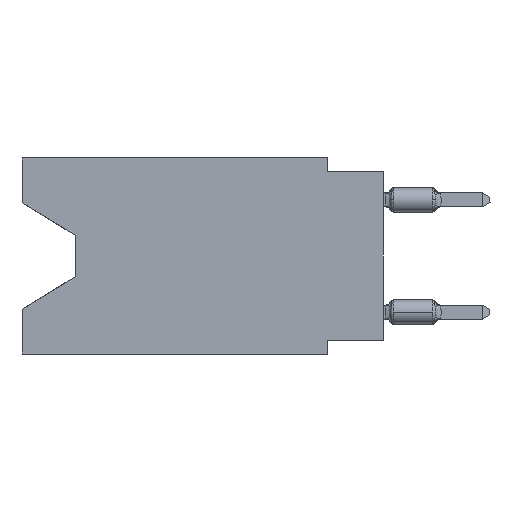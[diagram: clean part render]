
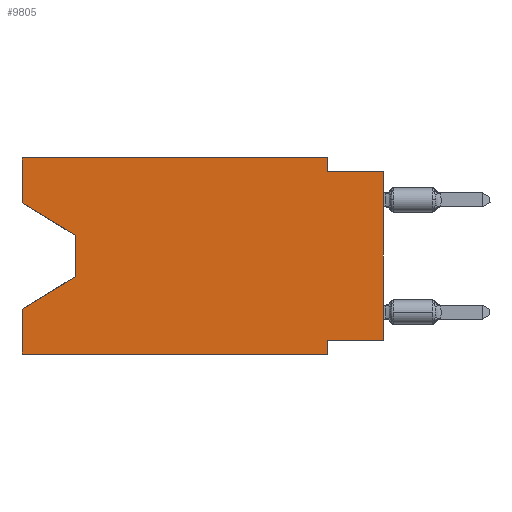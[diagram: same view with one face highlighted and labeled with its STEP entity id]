
A CAD part, left-side view. The second image highlights one B-rep face of the part: STEP entity #9805.
In plain terms, the highlighted planar face has unit normal (-1, 0, 0).
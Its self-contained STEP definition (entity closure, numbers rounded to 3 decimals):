
#19 = DIRECTION ( 'NONE',  ( 0., 0., 1. ) ) ;
#426 = EDGE_CURVE ( 'NONE', #23437, #9817, #18865, .T. ) ;
#440 = VECTOR ( 'NONE', #19, 1000. ) ;
#772 = EDGE_CURVE ( 'NONE', #21049, #9817, #8715, .T. ) ;
#2293 = ORIENTED_EDGE ( 'NONE', *, *, #16511, .F. ) ;
#2346 = ORIENTED_EDGE ( 'NONE', *, *, #4316, .F. ) ;
#2746 = DIRECTION ( 'NONE',  ( 0., 0., 1. ) ) ;
#3566 = ORIENTED_EDGE ( 'NONE', *, *, #21215, .T. ) ;
#3911 = PLANE ( 'NONE',  #6293 ) ;
#4005 = VERTEX_POINT ( 'NONE', #13388 ) ;
#4132 = CARTESIAN_POINT ( 'NONE',  ( 0., 16.383, -8.89 ) ) ;
#4316 = EDGE_CURVE ( 'NONE', #16762, #10100, #15087, .T. ) ;
#4825 = LINE ( 'NONE', #24658, #16931 ) ;
#5065 = CARTESIAN_POINT ( 'NONE',  ( 0., 2.54, -8.89 ) ) ;
#5200 = CARTESIAN_POINT ( 'NONE',  ( 0., 16.383, -8.89 ) ) ;
#5883 = CARTESIAN_POINT ( 'NONE',  ( 0., 0., -8.255 ) ) ;
#6238 = LINE ( 'NONE', #21960, #440 ) ;
#6293 = AXIS2_PLACEMENT_3D ( 'NONE', #12023, #8030, #9774 ) ;
#6436 = DIRECTION ( 'NONE',  ( 0., 0., -1. ) ) ;
#6662 = VERTEX_POINT ( 'NONE', #18724 ) ;
#6928 = CARTESIAN_POINT ( 'NONE',  ( 0., 2.54, 0. ) ) ;
#7099 = VERTEX_POINT ( 'NONE', #18822 ) ;
#7180 = VECTOR ( 'NONE', #24877, 1000. ) ;
#7308 = VERTEX_POINT ( 'NONE', #7891 ) ;
#7387 = ORIENTED_EDGE ( 'NONE', *, *, #16839, .F. ) ;
#7501 = CARTESIAN_POINT ( 'NONE',  ( 0., 16.383, 0. ) ) ;
#7617 = LINE ( 'NONE', #4132, #14617 ) ;
#7891 = CARTESIAN_POINT ( 'NONE',  ( 0., 16.383, 0. ) ) ;
#7902 = FACE_OUTER_BOUND ( 'NONE', #14123, .T. ) ;
#8030 = DIRECTION ( 'NONE',  ( 1., 0., 0. ) ) ;
#8398 = VECTOR ( 'NONE', #26050, 1000. ) ;
#8572 = CARTESIAN_POINT ( 'NONE',  ( 0., 16.383, 0. ) ) ;
#8715 = LINE ( 'NONE', #15461, #12296 ) ;
#8909 = LINE ( 'NONE', #6928, #7180 ) ;
#9039 = EDGE_CURVE ( 'NONE', #16762, #24889, #7617, .T. ) ;
#9488 = DIRECTION ( 'NONE',  ( 0., 1., 0. ) ) ;
#9670 = VECTOR ( 'NONE', #14174, 1000. ) ;
#9774 = DIRECTION ( 'NONE',  ( 0., 0., -1. ) ) ;
#9805 = ADVANCED_FACE ( 'NONE', ( #7902 ), #3911, .F. ) ;
#9817 = VERTEX_POINT ( 'NONE', #24267 ) ;
#10063 = CARTESIAN_POINT ( 'NONE',  ( 0., 0., -8.255 ) ) ;
#10100 = VERTEX_POINT ( 'NONE', #23066 ) ;
#10261 = ORIENTED_EDGE ( 'NONE', *, *, #9039, .T. ) ;
#10594 = VERTEX_POINT ( 'NONE', #24410 ) ;
#12023 = CARTESIAN_POINT ( 'NONE',  ( 0., 16.383, 0. ) ) ;
#12296 = VECTOR ( 'NONE', #2746, 1000. ) ;
#12490 = ORIENTED_EDGE ( 'NONE', *, *, #19169, .F. ) ;
#12650 = CARTESIAN_POINT ( 'NONE',  ( 0., 2.54, -0.635 ) ) ;
#12883 = ORIENTED_EDGE ( 'NONE', *, *, #21120, .T. ) ;
#13388 = CARTESIAN_POINT ( 'NONE',  ( 0., 16.383, -2.038 ) ) ;
#14115 = VECTOR ( 'NONE', #20959, 1000. ) ;
#14123 = EDGE_LOOP ( 'NONE', ( #3566, #20802, #12883, #2346, #10261, #7387, #25583, #17484, #17329, #12490, #2293, #18850 ) ) ;
#14174 = DIRECTION ( 'NONE',  ( 0., 0.855, -0.519 ) ) ;
#14333 = VECTOR ( 'NONE', #25090, 1000. ) ;
#14617 = VECTOR ( 'NONE', #16363, 1000. ) ;
#15087 = LINE ( 'NONE', #8572, #14115 ) ;
#15461 = CARTESIAN_POINT ( 'NONE',  ( 0., 0., 0. ) ) ;
#15661 = VECTOR ( 'NONE', #19261, 1000. ) ;
#15876 = LINE ( 'NONE', #5883, #24887 ) ;
#16363 = DIRECTION ( 'NONE',  ( 0., -1., 0. ) ) ;
#16511 = EDGE_CURVE ( 'NONE', #7308, #24226, #22123, .T. ) ;
#16700 = CARTESIAN_POINT ( 'NONE',  ( 0., 16.383, -2.038 ) ) ;
#16762 = VERTEX_POINT ( 'NONE', #5200 ) ;
#16839 = EDGE_CURVE ( 'NONE', #6662, #24889, #17931, .T. ) ;
#16931 = VECTOR ( 'NONE', #6436, 1000. ) ;
#16964 = LINE ( 'NONE', #16700, #14333 ) ;
#17329 = ORIENTED_EDGE ( 'NONE', *, *, #426, .F. ) ;
#17484 = ORIENTED_EDGE ( 'NONE', *, *, #772, .T. ) ;
#17634 = EDGE_CURVE ( 'NONE', #21049, #6662, #15876, .T. ) ;
#17727 = VECTOR ( 'NONE', #20120, 1000. ) ;
#17782 = CARTESIAN_POINT ( 'NONE',  ( 0., 13.97, -5.385 ) ) ;
#17802 = CARTESIAN_POINT ( 'NONE',  ( 0., 2.54, -8.89 ) ) ;
#17931 = LINE ( 'NONE', #17802, #8398 ) ;
#18724 = CARTESIAN_POINT ( 'NONE',  ( 0., 2.54, -8.255 ) ) ;
#18735 = CARTESIAN_POINT ( 'NONE',  ( 0., 0., -0.635 ) ) ;
#18822 = CARTESIAN_POINT ( 'NONE',  ( 0., 13.97, -3.505 ) ) ;
#18850 = ORIENTED_EDGE ( 'NONE', *, *, #24958, .F. ) ;
#18865 = LINE ( 'NONE', #18735, #15661 ) ;
#19169 = EDGE_CURVE ( 'NONE', #24226, #23437, #8909, .T. ) ;
#19261 = DIRECTION ( 'NONE',  ( 0., -1., 0. ) ) ;
#20120 = DIRECTION ( 'NONE',  ( 0., -1., 0. ) ) ;
#20170 = LINE ( 'NONE', #17782, #9670 ) ;
#20802 = ORIENTED_EDGE ( 'NONE', *, *, #23081, .T. ) ;
#20959 = DIRECTION ( 'NONE',  ( 0., 0., 1. ) ) ;
#21049 = VERTEX_POINT ( 'NONE', #10063 ) ;
#21120 = EDGE_CURVE ( 'NONE', #10594, #10100, #20170, .T. ) ;
#21215 = EDGE_CURVE ( 'NONE', #4005, #7099, #16964, .T. ) ;
#21541 = CARTESIAN_POINT ( 'NONE',  ( 0., 2.54, 0. ) ) ;
#21960 = CARTESIAN_POINT ( 'NONE',  ( 0., 16.383, 0. ) ) ;
#22123 = LINE ( 'NONE', #7501, #17727 ) ;
#23066 = CARTESIAN_POINT ( 'NONE',  ( 0., 16.383, -6.852 ) ) ;
#23081 = EDGE_CURVE ( 'NONE', #7099, #10594, #4825, .T. ) ;
#23437 = VERTEX_POINT ( 'NONE', #12650 ) ;
#24226 = VERTEX_POINT ( 'NONE', #21541 ) ;
#24267 = CARTESIAN_POINT ( 'NONE',  ( 0., 0., -0.635 ) ) ;
#24410 = CARTESIAN_POINT ( 'NONE',  ( 0., 13.97, -5.385 ) ) ;
#24658 = CARTESIAN_POINT ( 'NONE',  ( 0., 13.97, -3.505 ) ) ;
#24877 = DIRECTION ( 'NONE',  ( 0., 0., -1. ) ) ;
#24887 = VECTOR ( 'NONE', #9488, 1000. ) ;
#24889 = VERTEX_POINT ( 'NONE', #5065 ) ;
#24958 = EDGE_CURVE ( 'NONE', #4005, #7308, #6238, .T. ) ;
#25090 = DIRECTION ( 'NONE',  ( 0., -0.855, -0.519 ) ) ;
#25583 = ORIENTED_EDGE ( 'NONE', *, *, #17634, .F. ) ;
#26050 = DIRECTION ( 'NONE',  ( 0., 0., -1. ) ) ;
